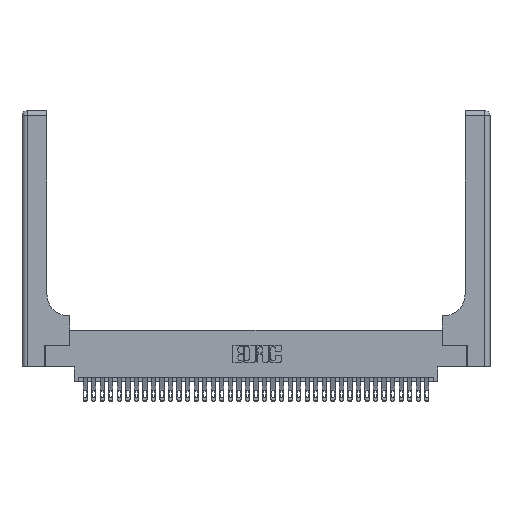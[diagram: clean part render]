
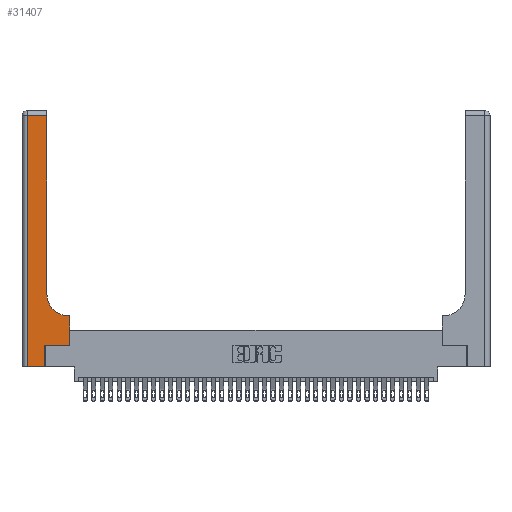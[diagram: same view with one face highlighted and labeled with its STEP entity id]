
A CAD part, top view. The second image highlights one B-rep face of the part: STEP entity #31407.
In plain terms, the highlighted planar face has unit normal (0, 0, 1).
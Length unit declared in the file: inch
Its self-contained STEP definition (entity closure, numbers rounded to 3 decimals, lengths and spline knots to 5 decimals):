
#140 = CARTESIAN_POINT ( 'NONE',  ( 0.2915, 0.6, 0.37 ) ) ;
#1457 = ORIENTED_EDGE ( 'NONE', *, *, #2500, .T. ) ;
#2500 = EDGE_CURVE ( 'NONE', #2860, #26628, #27736, .T. ) ;
#2860 = VERTEX_POINT ( 'NONE', #12225 ) ;
#2976 = DIRECTION ( 'NONE',  ( 0., 0., -1. ) ) ;
#3198 = CARTESIAN_POINT ( 'NONE',  ( 0.2915, 2.94, 0.37 ) ) ;
#3211 = CARTESIAN_POINT ( 'NONE',  ( 0., 0., 0.37 ) ) ;
#3324 = LINE ( 'NONE', #27405, #21736 ) ;
#3507 = AXIS2_PLACEMENT_3D ( 'NONE', #14694, #2976, #12263 ) ;
#3642 = DIRECTION ( 'NONE',  ( 0., 1., 0. ) ) ;
#4111 = EDGE_CURVE ( 'NONE', #11795, #16912, #8010, .T. ) ;
#5028 = AXIS2_PLACEMENT_3D ( 'NONE', #19814, #34602, #25624 ) ;
#5843 = DIRECTION ( 'NONE',  ( 0., -1., 0. ) ) ;
#5957 = DIRECTION ( 'NONE',  ( -1., 0., 0. ) ) ;
#6101 = LINE ( 'NONE', #27033, #36326 ) ;
#6560 = ORIENTED_EDGE ( 'NONE', *, *, #18244, .T. ) ;
#6690 = EDGE_CURVE ( 'NONE', #26628, #32918, #3324, .T. ) ;
#7699 = VECTOR ( 'NONE', #26997, 39.37008 ) ;
#8010 = LINE ( 'NONE', #10785, #24561 ) ;
#8402 = VECTOR ( 'NONE', #5957, 39.37008 ) ;
#8857 = VERTEX_POINT ( 'NONE', #19052 ) ;
#9007 = ORIENTED_EDGE ( 'NONE', *, *, #33339, .T. ) ;
#10249 = LINE ( 'NONE', #140, #8402 ) ;
#10785 = CARTESIAN_POINT ( 'NONE',  ( 0.2915, 3., 0.37 ) ) ;
#11795 = VERTEX_POINT ( 'NONE', #36251 ) ;
#12050 = ORIENTED_EDGE ( 'NONE', *, *, #24718, .T. ) ;
#12225 = CARTESIAN_POINT ( 'NONE',  ( 0.269, 0.25, 0.37 ) ) ;
#12263 = DIRECTION ( 'NONE',  ( -1., 0., 0. ) ) ;
#12480 = DIRECTION ( 'NONE',  ( 1., 0., 0. ) ) ;
#12488 = EDGE_LOOP ( 'NONE', ( #21125, #29741, #12050, #9007, #6560, #1457, #21425, #32788, #21129 ) ) ;
#12930 = CARTESIAN_POINT ( 'NONE',  ( 0., 2.94, 0.37 ) ) ;
#13251 = DIRECTION ( 'NONE',  ( 0., 1., 0. ) ) ;
#14694 = CARTESIAN_POINT ( 'NONE',  ( 0., 3., 0.37 ) ) ;
#14765 = CARTESIAN_POINT ( 'NONE',  ( 0.06, 2.94, 0.37 ) ) ;
#16359 = CARTESIAN_POINT ( 'NONE',  ( 0.5585, 0.6, 0.37 ) ) ;
#16912 = VERTEX_POINT ( 'NONE', #3198 ) ;
#17613 = PLANE ( 'NONE',  #3507 ) ;
#18045 = EDGE_CURVE ( 'NONE', #32918, #35173, #10249, .T. ) ;
#18244 = EDGE_CURVE ( 'NONE', #36232, #2860, #6101, .T. ) ;
#19052 = CARTESIAN_POINT ( 'NONE',  ( 0.06, 0., 0.37 ) ) ;
#19814 = CARTESIAN_POINT ( 'NONE',  ( 0.5415, 0.85, 0.37 ) ) ;
#20115 = CARTESIAN_POINT ( 'NONE',  ( 0.06, 3., 0.37 ) ) ;
#20697 = CARTESIAN_POINT ( 'NONE',  ( 0.269, 0., 0.37 ) ) ;
#21125 = ORIENTED_EDGE ( 'NONE', *, *, #4111, .T. ) ;
#21129 = ORIENTED_EDGE ( 'NONE', *, *, #22111, .T. ) ;
#21425 = ORIENTED_EDGE ( 'NONE', *, *, #6690, .T. ) ;
#21736 = VECTOR ( 'NONE', #24716, 39.37008 ) ;
#22111 = EDGE_CURVE ( 'NONE', #35173, #11795, #27690, .T. ) ;
#22866 = VECTOR ( 'NONE', #5843, 39.37008 ) ;
#24561 = VECTOR ( 'NONE', #13251, 39.37008 ) ;
#24716 = DIRECTION ( 'NONE',  ( 0., 1., 0. ) ) ;
#24718 = EDGE_CURVE ( 'NONE', #25841, #8857, #25652, .T. ) ;
#25121 = DIRECTION ( 'NONE',  ( -1., 0., 0. ) ) ;
#25624 = DIRECTION ( 'NONE',  ( 1., 0., 0. ) ) ;
#25652 = LINE ( 'NONE', #20115, #22866 ) ;
#25841 = VERTEX_POINT ( 'NONE', #14765 ) ;
#26628 = VERTEX_POINT ( 'NONE', #30251 ) ;
#26716 = CARTESIAN_POINT ( 'NONE',  ( 0.269, 0.25, 0.37 ) ) ;
#26997 = DIRECTION ( 'NONE',  ( 1., 0., 0. ) ) ;
#27033 = CARTESIAN_POINT ( 'NONE',  ( 0.269, 0., 0.37 ) ) ;
#27405 = CARTESIAN_POINT ( 'NONE',  ( 0.5585, 0.25, 0.37 ) ) ;
#27410 = EDGE_CURVE ( 'NONE', #16912, #25841, #36361, .T. ) ;
#27687 = CARTESIAN_POINT ( 'NONE',  ( 0.5415, 0.6, 0.37 ) ) ;
#27690 = CIRCLE ( 'NONE', #5028, 0.25 ) ;
#27736 = LINE ( 'NONE', #26716, #30452 ) ;
#28373 = FACE_OUTER_BOUND ( 'NONE', #12488, .T. ) ;
#29741 = ORIENTED_EDGE ( 'NONE', *, *, #27410, .T. ) ;
#30251 = CARTESIAN_POINT ( 'NONE',  ( 0.5585, 0.25, 0.37 ) ) ;
#30452 = VECTOR ( 'NONE', #12480, 39.37008 ) ;
#31090 = LINE ( 'NONE', #3211, #7699 ) ;
#31407 = ADVANCED_FACE ( 'NONE', ( #28373 ), #17613, .F. ) ;
#32788 = ORIENTED_EDGE ( 'NONE', *, *, #18045, .T. ) ;
#32918 = VERTEX_POINT ( 'NONE', #16359 ) ;
#33339 = EDGE_CURVE ( 'NONE', #8857, #36232, #31090, .T. ) ;
#33616 = VECTOR ( 'NONE', #25121, 39.37008 ) ;
#34602 = DIRECTION ( 'NONE',  ( 0., 0., -1. ) ) ;
#35173 = VERTEX_POINT ( 'NONE', #27687 ) ;
#36232 = VERTEX_POINT ( 'NONE', #20697 ) ;
#36251 = CARTESIAN_POINT ( 'NONE',  ( 0.2915, 0.85, 0.37 ) ) ;
#36326 = VECTOR ( 'NONE', #3642, 39.37008 ) ;
#36361 = LINE ( 'NONE', #12930, #33616 ) ;
